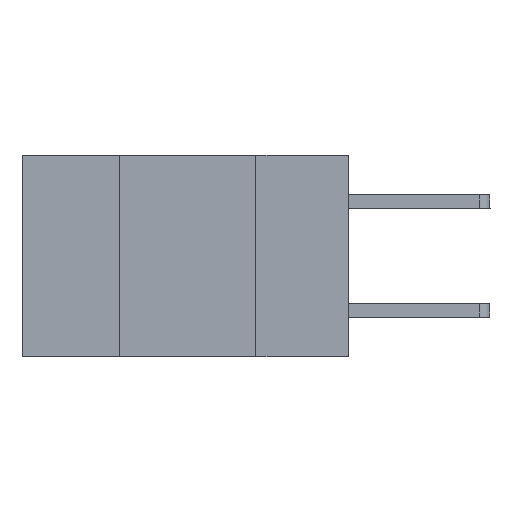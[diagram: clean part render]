
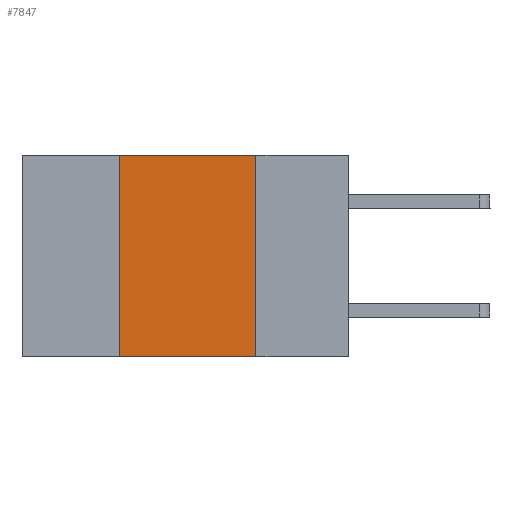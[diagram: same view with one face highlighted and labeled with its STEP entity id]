
A CAD part, left-side view. The second image highlights one B-rep face of the part: STEP entity #7847.
In plain terms, the highlighted planar face has unit normal (-1, 0, 0).
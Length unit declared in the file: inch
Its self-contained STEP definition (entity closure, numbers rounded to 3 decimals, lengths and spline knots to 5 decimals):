
#468 = VERTEX_POINT ( 'NONE', #2389 ) ;
#558 = CARTESIAN_POINT ( 'NONE',  ( 0., 0.42, -0.37 ) ) ;
#758 = VERTEX_POINT ( 'NONE', #10442 ) ;
#1303 = ORIENTED_EDGE ( 'NONE', *, *, #2255, .F. ) ;
#1458 = LINE ( 'NONE', #5625, #10545 ) ;
#1605 = VECTOR ( 'NONE', #4205, 39.37008 ) ;
#2255 = EDGE_CURVE ( 'NONE', #7428, #758, #9936, .T. ) ;
#2320 = EDGE_CURVE ( 'NONE', #7428, #468, #4975, .T. ) ;
#2343 = DIRECTION ( 'NONE',  ( 0., 0., 1. ) ) ;
#2389 = CARTESIAN_POINT ( 'NONE',  ( 0., 0.17, -0.37 ) ) ;
#2424 = VERTEX_POINT ( 'NONE', #6103 ) ;
#3512 = CARTESIAN_POINT ( 'NONE',  ( 0., 0.6, -0.37 ) ) ;
#3881 = DIRECTION ( 'NONE',  ( 0., -1., 0. ) ) ;
#4018 = LINE ( 'NONE', #7317, #6389 ) ;
#4205 = DIRECTION ( 'NONE',  ( 0., -1., 0. ) ) ;
#4208 = AXIS2_PLACEMENT_3D ( 'NONE', #6277, #7832, #9517 ) ;
#4481 = ORIENTED_EDGE ( 'NONE', *, *, #5356, .F. ) ;
#4975 = LINE ( 'NONE', #3512, #1605 ) ;
#5356 = EDGE_CURVE ( 'NONE', #2424, #468, #4018, .T. ) ;
#5476 = PLANE ( 'NONE',  #4208 ) ;
#5553 = EDGE_LOOP ( 'NONE', ( #4481, #7120, #1303, #10170 ) ) ;
#5625 = CARTESIAN_POINT ( 'NONE',  ( 0., 0.6, 0. ) ) ;
#5837 = CARTESIAN_POINT ( 'NONE',  ( 0., 0.42, 0. ) ) ;
#6103 = CARTESIAN_POINT ( 'NONE',  ( 0., 0.17, 0. ) ) ;
#6277 = CARTESIAN_POINT ( 'NONE',  ( 0., 0.6, 0. ) ) ;
#6389 = VECTOR ( 'NONE', #10618, 39.37008 ) ;
#7120 = ORIENTED_EDGE ( 'NONE', *, *, #9030, .F. ) ;
#7317 = CARTESIAN_POINT ( 'NONE',  ( 0., 0.17, 0. ) ) ;
#7428 = VERTEX_POINT ( 'NONE', #558 ) ;
#7832 = DIRECTION ( 'NONE',  ( 1., 0., 0. ) ) ;
#7847 = ADVANCED_FACE ( 'NONE', ( #8947 ), #5476, .F. ) ;
#8185 = VECTOR ( 'NONE', #2343, 39.37008 ) ;
#8947 = FACE_OUTER_BOUND ( 'NONE', #5553, .T. ) ;
#9030 = EDGE_CURVE ( 'NONE', #758, #2424, #1458, .T. ) ;
#9517 = DIRECTION ( 'NONE',  ( 0., 0., -1. ) ) ;
#9936 = LINE ( 'NONE', #5837, #8185 ) ;
#10170 = ORIENTED_EDGE ( 'NONE', *, *, #2320, .T. ) ;
#10442 = CARTESIAN_POINT ( 'NONE',  ( 0., 0.42, 0. ) ) ;
#10545 = VECTOR ( 'NONE', #3881, 39.37008 ) ;
#10618 = DIRECTION ( 'NONE',  ( 0., 0., -1. ) ) ;
